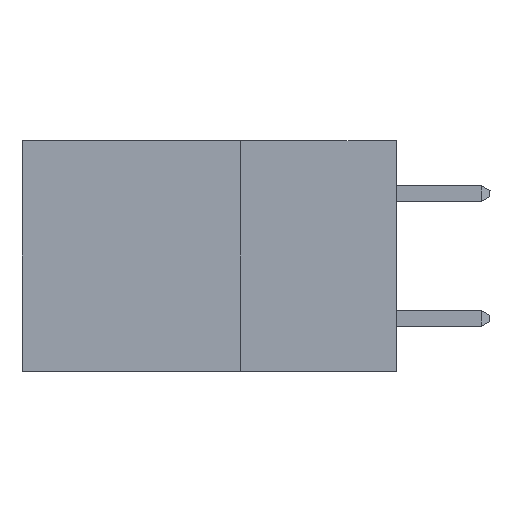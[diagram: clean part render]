
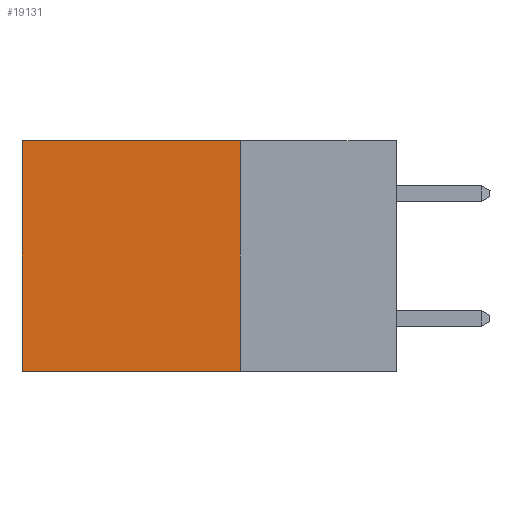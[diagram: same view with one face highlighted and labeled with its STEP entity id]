
A CAD part, left-side view. The second image highlights one B-rep face of the part: STEP entity #19131.
In plain terms, the highlighted planar face has unit normal (-1, 0, 0).
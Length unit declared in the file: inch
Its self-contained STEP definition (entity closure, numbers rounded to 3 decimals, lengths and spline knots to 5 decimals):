
#911 = DIRECTION ( 'NONE',  ( 1., 0., 0. ) ) ;
#1228 = EDGE_CURVE ( 'NONE', #17229, #23818, #8790, .T. ) ;
#2700 = VECTOR ( 'NONE', #5158, 39.37008 ) ;
#4270 = CARTESIAN_POINT ( 'NONE',  ( 0.298, 0.6, -0.37 ) ) ;
#5158 = DIRECTION ( 'NONE',  ( 0., 1., 0. ) ) ;
#5406 = EDGE_CURVE ( 'NONE', #13373, #21760, #16927, .T. ) ;
#5888 = CARTESIAN_POINT ( 'NONE',  ( 0.298, 0.6, 0. ) ) ;
#6615 = ORIENTED_EDGE ( 'NONE', *, *, #19268, .F. ) ;
#8790 = LINE ( 'NONE', #18612, #2700 ) ;
#8886 = FACE_OUTER_BOUND ( 'NONE', #11249, .T. ) ;
#10272 = CARTESIAN_POINT ( 'NONE',  ( 0.298, 0.6, 0. ) ) ;
#10895 = VECTOR ( 'NONE', #13853, 39.37008 ) ;
#11249 = EDGE_LOOP ( 'NONE', ( #23668, #24800, #6615, #19874 ) ) ;
#13128 = PLANE ( 'NONE',  #22626 ) ;
#13373 = VERTEX_POINT ( 'NONE', #13595 ) ;
#13399 = VECTOR ( 'NONE', #18306, 39.37008 ) ;
#13595 = CARTESIAN_POINT ( 'NONE',  ( 0.298, 0.25, 0. ) ) ;
#13832 = DIRECTION ( 'NONE',  ( 0., 0., -1. ) ) ;
#13853 = DIRECTION ( 'NONE',  ( 0., 1., 0. ) ) ;
#14478 = CARTESIAN_POINT ( 'NONE',  ( 0.298, 0.25, 0. ) ) ;
#15176 = DIRECTION ( 'NONE',  ( 0., 0., -1. ) ) ;
#15811 = CARTESIAN_POINT ( 'NONE',  ( 0.298, 0.25, 0. ) ) ;
#16472 = LINE ( 'NONE', #15811, #21150 ) ;
#16927 = LINE ( 'NONE', #14478, #10895 ) ;
#17166 = EDGE_CURVE ( 'NONE', #21760, #23818, #18803, .T. ) ;
#17229 = VERTEX_POINT ( 'NONE', #20481 ) ;
#18306 = DIRECTION ( 'NONE',  ( 0., 0., -1. ) ) ;
#18612 = CARTESIAN_POINT ( 'NONE',  ( 0.298, 0.25, -0.37 ) ) ;
#18803 = LINE ( 'NONE', #10272, #13399 ) ;
#19131 = ADVANCED_FACE ( 'NONE', ( #8886 ), #13128, .F. ) ;
#19148 = CARTESIAN_POINT ( 'NONE',  ( 0.298, 0.25, 0. ) ) ;
#19268 = EDGE_CURVE ( 'NONE', #13373, #17229, #16472, .T. ) ;
#19874 = ORIENTED_EDGE ( 'NONE', *, *, #5406, .T. ) ;
#20481 = CARTESIAN_POINT ( 'NONE',  ( 0.298, 0.25, -0.37 ) ) ;
#21150 = VECTOR ( 'NONE', #13832, 39.37008 ) ;
#21760 = VERTEX_POINT ( 'NONE', #5888 ) ;
#22626 = AXIS2_PLACEMENT_3D ( 'NONE', #19148, #911, #15176 ) ;
#23668 = ORIENTED_EDGE ( 'NONE', *, *, #17166, .T. ) ;
#23818 = VERTEX_POINT ( 'NONE', #4270 ) ;
#24800 = ORIENTED_EDGE ( 'NONE', *, *, #1228, .F. ) ;
